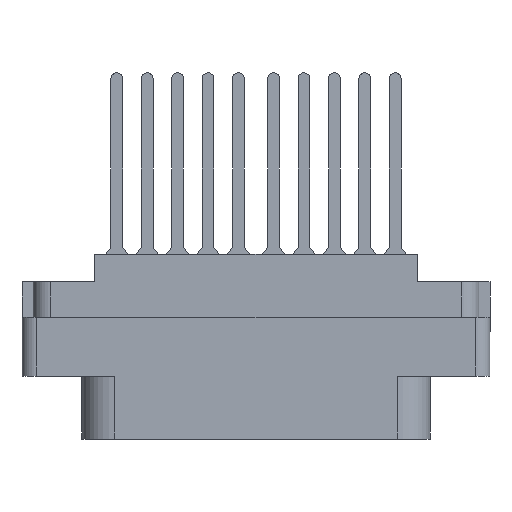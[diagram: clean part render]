
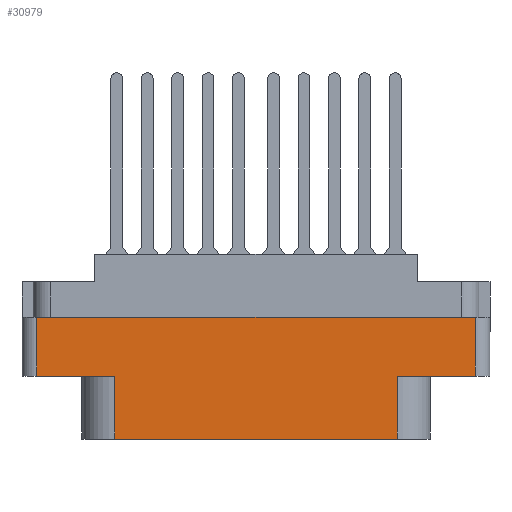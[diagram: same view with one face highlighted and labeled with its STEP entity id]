
A CAD part, front view. The second image highlights one B-rep face of the part: STEP entity #30979.
In plain terms, the highlighted planar face has unit normal (0, -1, 0).
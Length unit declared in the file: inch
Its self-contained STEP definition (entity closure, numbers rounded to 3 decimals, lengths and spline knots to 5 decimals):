
#175 = CARTESIAN_POINT ( 'NONE',  ( 0.938, -0.438, -0.52 ) ) ;
#619 = DIRECTION ( 'NONE',  ( 1., 0., 0. ) ) ;
#2214 = VECTOR ( 'NONE', #31072, 39.37008 ) ;
#2488 = DIRECTION ( 'NONE',  ( 1., 0., 0. ) ) ;
#3603 = CARTESIAN_POINT ( 'NONE',  ( -0.604, -0.438, -0.789 ) ) ;
#4443 = VECTOR ( 'NONE', #619, 39.37008 ) ;
#4716 = DIRECTION ( 'NONE',  ( 1., 0., 0. ) ) ;
#5060 = EDGE_CURVE ( 'NONE', #26526, #13174, #16760, .T. ) ;
#5504 = CARTESIAN_POINT ( 'NONE',  ( 0.604, -0.438, -0.52 ) ) ;
#5583 = EDGE_CURVE ( 'NONE', #13174, #21087, #23554, .T. ) ;
#5855 = VECTOR ( 'NONE', #7912, 39.37008 ) ;
#6066 = PLANE ( 'NONE',  #6170 ) ;
#6170 = AXIS2_PLACEMENT_3D ( 'NONE', #23224, #17506, #20410 ) ;
#6391 = DIRECTION ( 'NONE',  ( 0., 0., -1. ) ) ;
#7912 = DIRECTION ( 'NONE',  ( 0., 0., -1. ) ) ;
#8436 = EDGE_LOOP ( 'NONE', ( #34592, #8660, #35690, #16350, #18758, #23593, #8902, #30186 ) ) ;
#8660 = ORIENTED_EDGE ( 'NONE', *, *, #5060, .T. ) ;
#8902 = ORIENTED_EDGE ( 'NONE', *, *, #23121, .F. ) ;
#8970 = LINE ( 'NONE', #25335, #32685 ) ;
#9546 = CARTESIAN_POINT ( 'NONE',  ( 0., -0.438, -0.52 ) ) ;
#10683 = DIRECTION ( 'NONE',  ( 0., 0., 1. ) ) ;
#11199 = VECTOR ( 'NONE', #35955, 39.37008 ) ;
#13062 = CARTESIAN_POINT ( 'NONE',  ( 0.604, -0.438, -0.52 ) ) ;
#13174 = VERTEX_POINT ( 'NONE', #18567 ) ;
#13879 = CARTESIAN_POINT ( 'NONE',  ( -0.938, -0.438, -0.789 ) ) ;
#14125 = LINE ( 'NONE', #37344, #15464 ) ;
#14182 = CARTESIAN_POINT ( 'NONE',  ( -0.938, -0.438, -0.268 ) ) ;
#15426 = EDGE_CURVE ( 'NONE', #21087, #22052, #32819, .T. ) ;
#15464 = VECTOR ( 'NONE', #2488, 39.37008 ) ;
#15804 = VERTEX_POINT ( 'NONE', #175 ) ;
#16292 = CARTESIAN_POINT ( 'NONE',  ( 0., -0.438, -0.268 ) ) ;
#16350 = ORIENTED_EDGE ( 'NONE', *, *, #15426, .T. ) ;
#16432 = CARTESIAN_POINT ( 'NONE',  ( 0.604, -0.438, -0.789 ) ) ;
#16760 = LINE ( 'NONE', #13879, #5855 ) ;
#16883 = EDGE_CURVE ( 'NONE', #26526, #21547, #34564, .T. ) ;
#17506 = DIRECTION ( 'NONE',  ( 0., -1., 0. ) ) ;
#17762 = CARTESIAN_POINT ( 'NONE',  ( 0.938, -0.438, -0.268 ) ) ;
#18179 = VECTOR ( 'NONE', #6391, 39.37008 ) ;
#18567 = CARTESIAN_POINT ( 'NONE',  ( -0.938, -0.438, -0.52 ) ) ;
#18758 = ORIENTED_EDGE ( 'NONE', *, *, #35186, .T. ) ;
#20410 = DIRECTION ( 'NONE',  ( 0., 0., -1. ) ) ;
#21087 = VERTEX_POINT ( 'NONE', #36164 ) ;
#21547 = VERTEX_POINT ( 'NONE', #17762 ) ;
#22052 = VERTEX_POINT ( 'NONE', #23649 ) ;
#22184 = VECTOR ( 'NONE', #4716, 39.37008 ) ;
#23121 = EDGE_CURVE ( 'NONE', #15804, #36072, #28527, .T. ) ;
#23224 = CARTESIAN_POINT ( 'NONE',  ( -1., -0.438, -0.789 ) ) ;
#23524 = LINE ( 'NONE', #13062, #2214 ) ;
#23554 = LINE ( 'NONE', #23815, #4443 ) ;
#23593 = ORIENTED_EDGE ( 'NONE', *, *, #27638, .T. ) ;
#23649 = CARTESIAN_POINT ( 'NONE',  ( -0.604, -0.438, -0.789 ) ) ;
#23772 = FACE_OUTER_BOUND ( 'NONE', #8436, .T. ) ;
#23815 = CARTESIAN_POINT ( 'NONE',  ( 0., -0.438, -0.52 ) ) ;
#25335 = CARTESIAN_POINT ( 'NONE',  ( 0.938, -0.438, -0.789 ) ) ;
#26526 = VERTEX_POINT ( 'NONE', #14182 ) ;
#27638 = EDGE_CURVE ( 'NONE', #32040, #36072, #23524, .T. ) ;
#28527 = LINE ( 'NONE', #9546, #11199 ) ;
#30186 = ORIENTED_EDGE ( 'NONE', *, *, #36997, .T. ) ;
#30979 = ADVANCED_FACE ( 'NONE', ( #23772 ), #6066, .T. ) ;
#31072 = DIRECTION ( 'NONE',  ( 0., 0., 1. ) ) ;
#32040 = VERTEX_POINT ( 'NONE', #16432 ) ;
#32685 = VECTOR ( 'NONE', #10683, 39.37008 ) ;
#32819 = LINE ( 'NONE', #3603, #18179 ) ;
#34564 = LINE ( 'NONE', #16292, #22184 ) ;
#34592 = ORIENTED_EDGE ( 'NONE', *, *, #16883, .F. ) ;
#35186 = EDGE_CURVE ( 'NONE', #22052, #32040, #14125, .T. ) ;
#35690 = ORIENTED_EDGE ( 'NONE', *, *, #5583, .T. ) ;
#35955 = DIRECTION ( 'NONE',  ( -1., 0., 0. ) ) ;
#36072 = VERTEX_POINT ( 'NONE', #5504 ) ;
#36164 = CARTESIAN_POINT ( 'NONE',  ( -0.604, -0.438, -0.52 ) ) ;
#36997 = EDGE_CURVE ( 'NONE', #15804, #21547, #8970, .T. ) ;
#37344 = CARTESIAN_POINT ( 'NONE',  ( -1., -0.438, -0.789 ) ) ;
